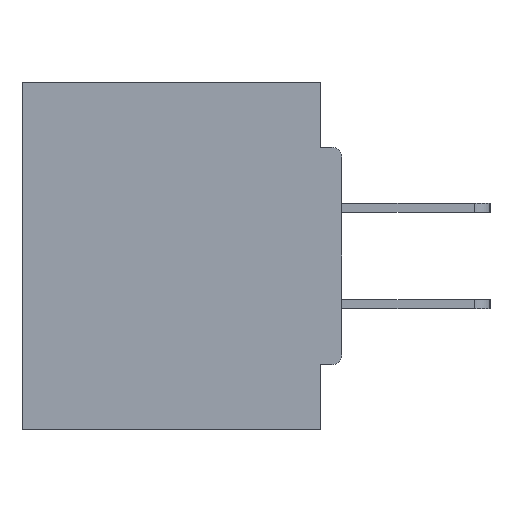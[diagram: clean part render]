
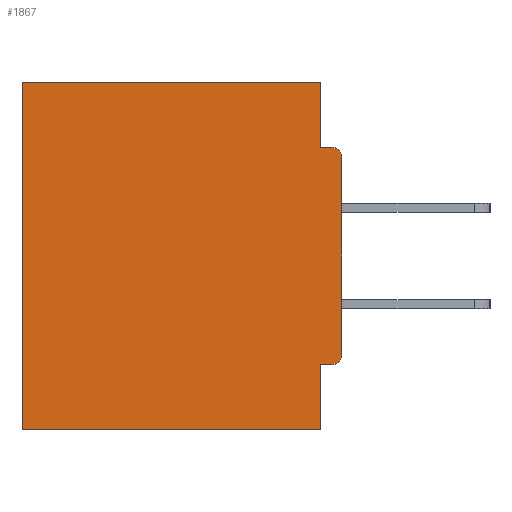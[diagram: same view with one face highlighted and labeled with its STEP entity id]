
A CAD part, left-side view. The second image highlights one B-rep face of the part: STEP entity #1867.
In plain terms, the highlighted planar face has unit normal (-1, 0, 0).
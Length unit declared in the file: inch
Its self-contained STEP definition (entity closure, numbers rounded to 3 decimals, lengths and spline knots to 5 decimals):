
#354 = EDGE_CURVE ( 'NONE', #24177, #1882, #18326, .T. ) ;
#783 = VERTEX_POINT ( 'NONE', #31438 ) ;
#1619 = CARTESIAN_POINT ( 'NONE',  ( 0.298, 0.031, -0.4065 ) ) ;
#1867 = ADVANCED_FACE ( 'NONE', ( #25502 ), #19368, .F. ) ;
#1882 = VERTEX_POINT ( 'NONE', #1937 ) ;
#1937 = CARTESIAN_POINT ( 'NONE',  ( 0.298, 0.46, -0.5 ) ) ;
#2265 = VERTEX_POINT ( 'NONE', #12105 ) ;
#2398 = CARTESIAN_POINT ( 'NONE',  ( 0.298, 0.015, -0.3915 ) ) ;
#3262 = CARTESIAN_POINT ( 'NONE',  ( 0.298, 0.46, 0. ) ) ;
#3399 = DIRECTION ( 'NONE',  ( 0., 0., -1. ) ) ;
#3422 = LINE ( 'NONE', #20933, #6293 ) ;
#3593 = ORIENTED_EDGE ( 'NONE', *, *, #20247, .T. ) ;
#5417 = EDGE_CURVE ( 'NONE', #21279, #783, #3422, .T. ) ;
#6293 = VECTOR ( 'NONE', #15867, 39.37008 ) ;
#7024 = CARTESIAN_POINT ( 'NONE',  ( 0.298, 0., 0. ) ) ;
#7699 = ORIENTED_EDGE ( 'NONE', *, *, #26639, .F. ) ;
#8184 = ORIENTED_EDGE ( 'NONE', *, *, #32885, .T. ) ;
#9391 = DIRECTION ( 'NONE',  ( -1., 0., 0. ) ) ;
#9640 = CARTESIAN_POINT ( 'NONE',  ( 0.298, 0.031, -0.5 ) ) ;
#9797 = EDGE_CURVE ( 'NONE', #2265, #22190, #26188, .T. ) ;
#9804 = DIRECTION ( 'NONE',  ( 0., 0., -1. ) ) ;
#10016 = EDGE_CURVE ( 'NONE', #12334, #31279, #27394, .T. ) ;
#10305 = CARTESIAN_POINT ( 'NONE',  ( 0.298, 0.46, 0. ) ) ;
#10352 = CARTESIAN_POINT ( 'NONE',  ( 0.298, 0., -0.0935 ) ) ;
#10463 = CARTESIAN_POINT ( 'NONE',  ( 0.298, 0., -0.1085 ) ) ;
#11039 = CARTESIAN_POINT ( 'NONE',  ( 0.298, 0., -0.4065 ) ) ;
#11829 = CARTESIAN_POINT ( 'NONE',  ( 0.298, 0.015, -0.1085 ) ) ;
#12047 = CARTESIAN_POINT ( 'NONE',  ( 0.298, 0.031, -0.5 ) ) ;
#12105 = CARTESIAN_POINT ( 'NONE',  ( 0.298, 0.015, -0.4065 ) ) ;
#12334 = VERTEX_POINT ( 'NONE', #29523 ) ;
#12485 = CIRCLE ( 'NONE', #29468, 0.015 ) ;
#13632 = VECTOR ( 'NONE', #23960, 39.37008 ) ;
#14816 = EDGE_CURVE ( 'NONE', #22190, #24177, #29400, .T. ) ;
#15867 = DIRECTION ( 'NONE',  ( 0., 0., -1. ) ) ;
#15965 = CARTESIAN_POINT ( 'NONE',  ( 0.298, 0.015, -0.0935 ) ) ;
#16630 = ORIENTED_EDGE ( 'NONE', *, *, #10016, .F. ) ;
#17377 = DIRECTION ( 'NONE',  ( 0., 1., 0. ) ) ;
#17497 = EDGE_CURVE ( 'NONE', #21279, #31279, #21402, .T. ) ;
#17603 = EDGE_CURVE ( 'NONE', #2265, #783, #12485, .T. ) ;
#17964 = VERTEX_POINT ( 'NONE', #10305 ) ;
#18129 = DIRECTION ( 'NONE',  ( 0., -1., 0. ) ) ;
#18326 = LINE ( 'NONE', #29580, #26860 ) ;
#18566 = CARTESIAN_POINT ( 'NONE',  ( 0.298, 0.031, -0.5 ) ) ;
#19272 = VECTOR ( 'NONE', #31908, 39.37008 ) ;
#19368 = PLANE ( 'NONE',  #29493 ) ;
#19443 = CARTESIAN_POINT ( 'NONE',  ( 0.298, 0.031, 0. ) ) ;
#19631 = ORIENTED_EDGE ( 'NONE', *, *, #5417, .F. ) ;
#19687 = DIRECTION ( 'NONE',  ( 0., 0., -1. ) ) ;
#20098 = LINE ( 'NONE', #3262, #13632 ) ;
#20247 = EDGE_CURVE ( 'NONE', #27695, #17964, #26957, .T. ) ;
#20482 = VECTOR ( 'NONE', #18129, 39.37008 ) ;
#20587 = ORIENTED_EDGE ( 'NONE', *, *, #354, .F. ) ;
#20933 = CARTESIAN_POINT ( 'NONE',  ( 0.298, 0., 0. ) ) ;
#21279 = VERTEX_POINT ( 'NONE', #10463 ) ;
#21402 = CIRCLE ( 'NONE', #31220, 0.015 ) ;
#22190 = VERTEX_POINT ( 'NONE', #1619 ) ;
#22478 = VECTOR ( 'NONE', #19687, 39.37008 ) ;
#23376 = ORIENTED_EDGE ( 'NONE', *, *, #14816, .F. ) ;
#23944 = CARTESIAN_POINT ( 'NONE',  ( 0.298, 0., 0. ) ) ;
#23960 = DIRECTION ( 'NONE',  ( 0., 0., -1. ) ) ;
#24094 = VECTOR ( 'NONE', #3399, 39.37008 ) ;
#24177 = VERTEX_POINT ( 'NONE', #18566 ) ;
#25285 = LINE ( 'NONE', #12047, #24094 ) ;
#25502 = FACE_OUTER_BOUND ( 'NONE', #28642, .T. ) ;
#26147 = ORIENTED_EDGE ( 'NONE', *, *, #17497, .T. ) ;
#26188 = LINE ( 'NONE', #11039, #19272 ) ;
#26639 = EDGE_CURVE ( 'NONE', #27695, #12334, #25285, .T. ) ;
#26860 = VECTOR ( 'NONE', #32534, 39.37008 ) ;
#26957 = LINE ( 'NONE', #7024, #33066 ) ;
#27394 = LINE ( 'NONE', #10352, #20482 ) ;
#27473 = ORIENTED_EDGE ( 'NONE', *, *, #9797, .F. ) ;
#27695 = VERTEX_POINT ( 'NONE', #19443 ) ;
#28054 = DIRECTION ( 'NONE',  ( -1., 0., 0. ) ) ;
#28642 = EDGE_LOOP ( 'NONE', ( #26147, #16630, #7699, #3593, #8184, #20587, #23376, #27473, #31118, #19631 ) ) ;
#29400 = LINE ( 'NONE', #9640, #22478 ) ;
#29468 = AXIS2_PLACEMENT_3D ( 'NONE', #2398, #28054, #33182 ) ;
#29493 = AXIS2_PLACEMENT_3D ( 'NONE', #23944, #32939, #9804 ) ;
#29523 = CARTESIAN_POINT ( 'NONE',  ( 0.298, 0.031, -0.0935 ) ) ;
#29580 = CARTESIAN_POINT ( 'NONE',  ( 0.298, 0., -0.5 ) ) ;
#29889 = DIRECTION ( 'NONE',  ( 0., 0., -1. ) ) ;
#31118 = ORIENTED_EDGE ( 'NONE', *, *, #17603, .T. ) ;
#31220 = AXIS2_PLACEMENT_3D ( 'NONE', #11829, #9391, #29889 ) ;
#31279 = VERTEX_POINT ( 'NONE', #15965 ) ;
#31438 = CARTESIAN_POINT ( 'NONE',  ( 0.298, 0., -0.3915 ) ) ;
#31908 = DIRECTION ( 'NONE',  ( 0., 1., 0. ) ) ;
#32534 = DIRECTION ( 'NONE',  ( 0., 1., 0. ) ) ;
#32885 = EDGE_CURVE ( 'NONE', #17964, #1882, #20098, .T. ) ;
#32939 = DIRECTION ( 'NONE',  ( 1., 0., 0. ) ) ;
#33066 = VECTOR ( 'NONE', #17377, 39.37008 ) ;
#33182 = DIRECTION ( 'NONE',  ( 0., 0., -1. ) ) ;
